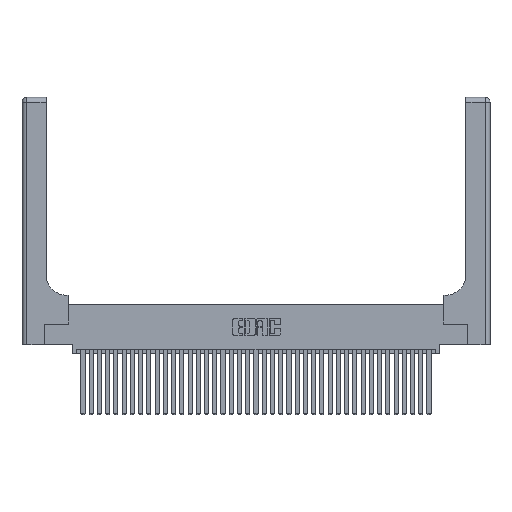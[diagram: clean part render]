
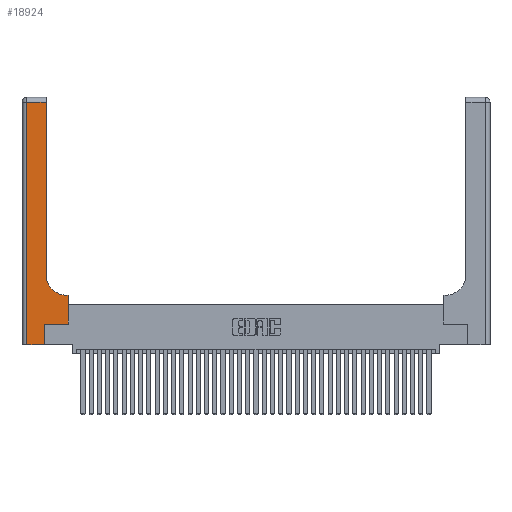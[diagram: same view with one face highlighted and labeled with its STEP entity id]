
A CAD part, top view. The second image highlights one B-rep face of the part: STEP entity #18924.
In plain terms, the highlighted planar face has unit normal (0, 0, 1).
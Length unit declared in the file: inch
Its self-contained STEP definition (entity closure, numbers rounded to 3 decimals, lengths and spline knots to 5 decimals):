
#1082 = CIRCLE ( 'NONE', #12042, 0.25 ) ;
#1106 = VECTOR ( 'NONE', #1310, 39.37008 ) ;
#1152 = VERTEX_POINT ( 'NONE', #11369 ) ;
#1310 = DIRECTION ( 'NONE',  ( 0., 1., 0. ) ) ;
#1654 = DIRECTION ( 'NONE',  ( 1., 0., 0. ) ) ;
#1861 = LINE ( 'NONE', #9353, #32780 ) ;
#1955 = VERTEX_POINT ( 'NONE', #11039 ) ;
#2606 = CARTESIAN_POINT ( 'NONE',  ( 0.2915, 0.85, 0.37 ) ) ;
#3056 = EDGE_CURVE ( 'NONE', #24935, #1955, #34858, .T. ) ;
#3241 = CARTESIAN_POINT ( 'NONE',  ( 0., 2.94, 0.37 ) ) ;
#3988 = EDGE_CURVE ( 'NONE', #30681, #17650, #29760, .T. ) ;
#4156 = DIRECTION ( 'NONE',  ( 0., 0., -1. ) ) ;
#4857 = DIRECTION ( 'NONE',  ( 0., -1., 0. ) ) ;
#5047 = EDGE_CURVE ( 'NONE', #25702, #24935, #1082, .T. ) ;
#6291 = ORIENTED_EDGE ( 'NONE', *, *, #38616, .T. ) ;
#6356 = CARTESIAN_POINT ( 'NONE',  ( 0.5415, 0.6, 0.37 ) ) ;
#6712 = CARTESIAN_POINT ( 'NONE',  ( 0.2915, 3., 0.37 ) ) ;
#7250 = VERTEX_POINT ( 'NONE', #36165 ) ;
#8044 = LINE ( 'NONE', #14747, #30962 ) ;
#8124 = CARTESIAN_POINT ( 'NONE',  ( 0.06, 0., 0.37 ) ) ;
#9353 = CARTESIAN_POINT ( 'NONE',  ( 0.269, 0.25, 0.37 ) ) ;
#9937 = VECTOR ( 'NONE', #10127, 39.37008 ) ;
#10015 = EDGE_CURVE ( 'NONE', #1955, #19769, #25226, .T. ) ;
#10127 = DIRECTION ( 'NONE',  ( -1., 0., 0. ) ) ;
#10218 = DIRECTION ( 'NONE',  ( -1., 0., 0. ) ) ;
#11039 = CARTESIAN_POINT ( 'NONE',  ( 0.2915, 2.94, 0.37 ) ) ;
#11369 = CARTESIAN_POINT ( 'NONE',  ( 0.5585, 0.25, 0.37 ) ) ;
#12042 = AXIS2_PLACEMENT_3D ( 'NONE', #34122, #19507, #1654 ) ;
#12709 = LINE ( 'NONE', #34187, #9937 ) ;
#13654 = CARTESIAN_POINT ( 'NONE',  ( 0.269, 0., 0.37 ) ) ;
#13658 = CARTESIAN_POINT ( 'NONE',  ( 0.06, 2.94, 0.37 ) ) ;
#14102 = ORIENTED_EDGE ( 'NONE', *, *, #10015, .T. ) ;
#14585 = EDGE_LOOP ( 'NONE', ( #24551, #14102, #6291, #32335, #32591, #36294, #20049, #21997, #29982 ) ) ;
#14747 = CARTESIAN_POINT ( 'NONE',  ( 0., 0., 0.37 ) ) ;
#15148 = FACE_OUTER_BOUND ( 'NONE', #14585, .T. ) ;
#17650 = VERTEX_POINT ( 'NONE', #22541 ) ;
#18515 = DIRECTION ( 'NONE',  ( 1., 0., 0. ) ) ;
#18924 = ADVANCED_FACE ( 'NONE', ( #15148 ), #37038, .F. ) ;
#19073 = VECTOR ( 'NONE', #32717, 39.37008 ) ;
#19507 = DIRECTION ( 'NONE',  ( 0., 0., -1. ) ) ;
#19769 = VERTEX_POINT ( 'NONE', #13658 ) ;
#20049 = ORIENTED_EDGE ( 'NONE', *, *, #34863, .T. ) ;
#20402 = VECTOR ( 'NONE', #36437, 39.37008 ) ;
#21047 = VERTEX_POINT ( 'NONE', #8124 ) ;
#21891 = CARTESIAN_POINT ( 'NONE',  ( 0.269, 0., 0.37 ) ) ;
#21997 = ORIENTED_EDGE ( 'NONE', *, *, #32380, .T. ) ;
#22541 = CARTESIAN_POINT ( 'NONE',  ( 0.269, 0.25, 0.37 ) ) ;
#23772 = DIRECTION ( 'NONE',  ( 1., 0., 0. ) ) ;
#24551 = ORIENTED_EDGE ( 'NONE', *, *, #3056, .T. ) ;
#24935 = VERTEX_POINT ( 'NONE', #2606 ) ;
#25145 = LINE ( 'NONE', #33426, #20402 ) ;
#25226 = LINE ( 'NONE', #3241, #19073 ) ;
#25702 = VERTEX_POINT ( 'NONE', #6356 ) ;
#28121 = CARTESIAN_POINT ( 'NONE',  ( 0., 3., 0.37 ) ) ;
#29760 = LINE ( 'NONE', #21891, #33494 ) ;
#29982 = ORIENTED_EDGE ( 'NONE', *, *, #5047, .T. ) ;
#30327 = EDGE_CURVE ( 'NONE', #21047, #30681, #8044, .T. ) ;
#30681 = VERTEX_POINT ( 'NONE', #13654 ) ;
#30962 = VECTOR ( 'NONE', #23772, 39.37008 ) ;
#31482 = LINE ( 'NONE', #38076, #37548 ) ;
#32335 = ORIENTED_EDGE ( 'NONE', *, *, #30327, .T. ) ;
#32380 = EDGE_CURVE ( 'NONE', #7250, #25702, #12709, .T. ) ;
#32591 = ORIENTED_EDGE ( 'NONE', *, *, #3988, .T. ) ;
#32717 = DIRECTION ( 'NONE',  ( -1., 0., 0. ) ) ;
#32780 = VECTOR ( 'NONE', #18515, 39.37008 ) ;
#33398 = EDGE_CURVE ( 'NONE', #17650, #1152, #1861, .T. ) ;
#33426 = CARTESIAN_POINT ( 'NONE',  ( 0.5585, 0.25, 0.37 ) ) ;
#33494 = VECTOR ( 'NONE', #37015, 39.37008 ) ;
#34122 = CARTESIAN_POINT ( 'NONE',  ( 0.5415, 0.85, 0.37 ) ) ;
#34187 = CARTESIAN_POINT ( 'NONE',  ( 0.2915, 0.6, 0.37 ) ) ;
#34858 = LINE ( 'NONE', #6712, #1106 ) ;
#34863 = EDGE_CURVE ( 'NONE', #1152, #7250, #25145, .T. ) ;
#36165 = CARTESIAN_POINT ( 'NONE',  ( 0.5585, 0.6, 0.37 ) ) ;
#36294 = ORIENTED_EDGE ( 'NONE', *, *, #33398, .T. ) ;
#36437 = DIRECTION ( 'NONE',  ( 0., 1., 0. ) ) ;
#37015 = DIRECTION ( 'NONE',  ( 0., 1., 0. ) ) ;
#37038 = PLANE ( 'NONE',  #37134 ) ;
#37134 = AXIS2_PLACEMENT_3D ( 'NONE', #28121, #4156, #10218 ) ;
#37548 = VECTOR ( 'NONE', #4857, 39.37008 ) ;
#38076 = CARTESIAN_POINT ( 'NONE',  ( 0.06, 3., 0.37 ) ) ;
#38616 = EDGE_CURVE ( 'NONE', #19769, #21047, #31482, .T. ) ;
